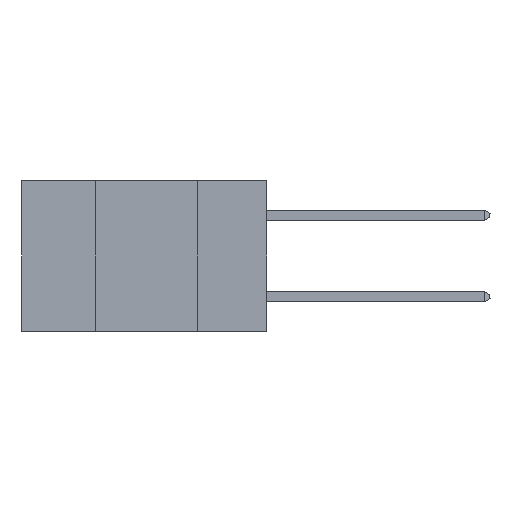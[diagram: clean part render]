
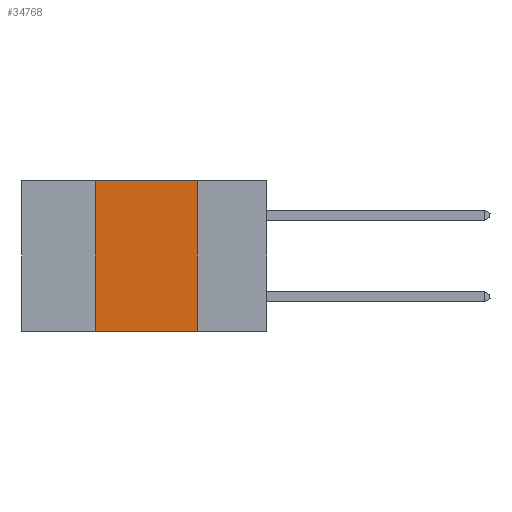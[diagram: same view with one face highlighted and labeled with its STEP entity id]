
A CAD part, left-side view. The second image highlights one B-rep face of the part: STEP entity #34768.
In plain terms, the highlighted planar face has unit normal (-1, 0, 0).
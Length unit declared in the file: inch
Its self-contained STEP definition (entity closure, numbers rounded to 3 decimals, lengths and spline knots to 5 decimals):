
#332 = EDGE_CURVE ( 'NONE', #38535, #31661, #2629, .T. ) ;
#2629 = LINE ( 'NONE', #15335, #34642 ) ;
#2676 = CARTESIAN_POINT ( 'NONE',  ( 0., 0.42, 0. ) ) ;
#3576 = DIRECTION ( 'NONE',  ( 0., 0., -1. ) ) ;
#4967 = VECTOR ( 'NONE', #8240, 39.37008 ) ;
#5674 = DIRECTION ( 'NONE',  ( 0., 0., 1. ) ) ;
#8240 = DIRECTION ( 'NONE',  ( 0., 0., -1. ) ) ;
#9499 = CARTESIAN_POINT ( 'NONE',  ( 0., 0.6, 0. ) ) ;
#9515 = EDGE_CURVE ( 'NONE', #9886, #15577, #9709, .T. ) ;
#9637 = PLANE ( 'NONE',  #29236 ) ;
#9709 = LINE ( 'NONE', #24388, #32260 ) ;
#9886 = VERTEX_POINT ( 'NONE', #26060 ) ;
#10375 = ORIENTED_EDGE ( 'NONE', *, *, #29789, .F. ) ;
#10759 = ORIENTED_EDGE ( 'NONE', *, *, #9515, .T. ) ;
#10961 = CARTESIAN_POINT ( 'NONE',  ( 0., 0.42, 0. ) ) ;
#12245 = EDGE_CURVE ( 'NONE', #9886, #38535, #22406, .T. ) ;
#12958 = LINE ( 'NONE', #14394, #4967 ) ;
#14131 = ORIENTED_EDGE ( 'NONE', *, *, #332, .F. ) ;
#14328 = VECTOR ( 'NONE', #5674, 39.37008 ) ;
#14394 = CARTESIAN_POINT ( 'NONE',  ( 0., 0.17, 0. ) ) ;
#15335 = CARTESIAN_POINT ( 'NONE',  ( 0., 0.6, 0. ) ) ;
#15577 = VERTEX_POINT ( 'NONE', #33708 ) ;
#15609 = DIRECTION ( 'NONE',  ( 0., -1., 0. ) ) ;
#22406 = LINE ( 'NONE', #2676, #14328 ) ;
#24254 = DIRECTION ( 'NONE',  ( 1., 0., 0. ) ) ;
#24388 = CARTESIAN_POINT ( 'NONE',  ( 0., 0.6, -0.37 ) ) ;
#25831 = ORIENTED_EDGE ( 'NONE', *, *, #12245, .F. ) ;
#26060 = CARTESIAN_POINT ( 'NONE',  ( 0., 0.42, -0.37 ) ) ;
#29236 = AXIS2_PLACEMENT_3D ( 'NONE', #9499, #24254, #3576 ) ;
#29789 = EDGE_CURVE ( 'NONE', #31661, #15577, #12958, .T. ) ;
#29993 = FACE_OUTER_BOUND ( 'NONE', #38086, .T. ) ;
#31661 = VERTEX_POINT ( 'NONE', #38258 ) ;
#32260 = VECTOR ( 'NONE', #33974, 39.37008 ) ;
#33708 = CARTESIAN_POINT ( 'NONE',  ( 0., 0.17, -0.37 ) ) ;
#33974 = DIRECTION ( 'NONE',  ( 0., -1., 0. ) ) ;
#34642 = VECTOR ( 'NONE', #15609, 39.37008 ) ;
#34768 = ADVANCED_FACE ( 'NONE', ( #29993 ), #9637, .F. ) ;
#38086 = EDGE_LOOP ( 'NONE', ( #10375, #14131, #25831, #10759 ) ) ;
#38258 = CARTESIAN_POINT ( 'NONE',  ( 0., 0.17, 0. ) ) ;
#38535 = VERTEX_POINT ( 'NONE', #10961 ) ;
